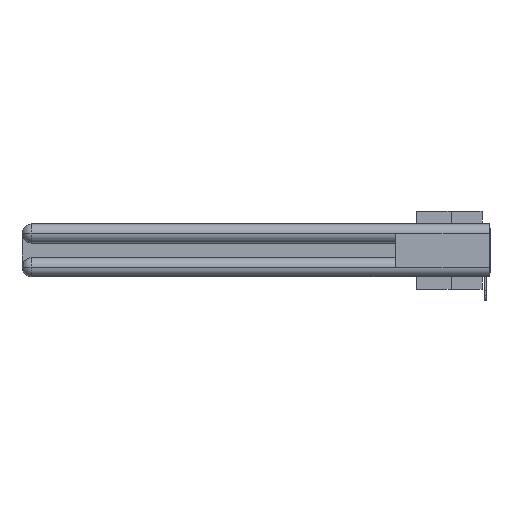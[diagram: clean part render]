
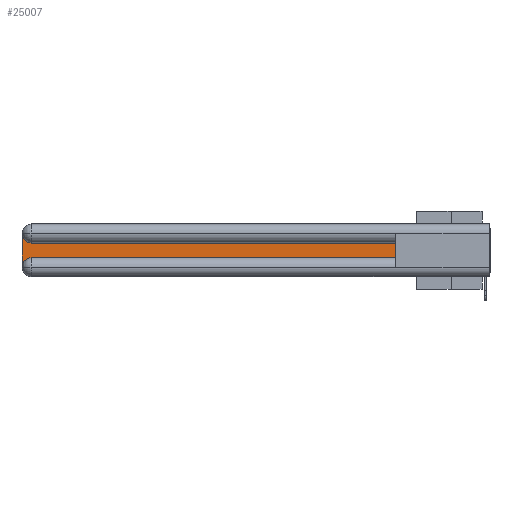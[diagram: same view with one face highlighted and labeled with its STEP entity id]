
A CAD part, left-side view. The second image highlights one B-rep face of the part: STEP entity #25007.
In plain terms, the highlighted planar face has unit normal (-1, 0, 0).
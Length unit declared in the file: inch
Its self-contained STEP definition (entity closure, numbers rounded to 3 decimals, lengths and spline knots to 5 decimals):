
#754 = VECTOR ( 'NONE', #11253, 39.37008 ) ;
#783 = CARTESIAN_POINT ( 'NONE',  ( 0.075, 2.94, -0.2775 ) ) ;
#1091 = DIRECTION ( 'NONE',  ( 1., 0., 0. ) ) ;
#2215 = CIRCLE ( 'NONE', #4742, 0.06 ) ;
#2642 = DIRECTION ( 'NONE',  ( 0., 0., -1. ) ) ;
#4244 = CARTESIAN_POINT ( 'NONE',  ( 0.075, 3., -0.2775 ) ) ;
#4317 = AXIS2_PLACEMENT_3D ( 'NONE', #28802, #22322, #26256 ) ;
#4633 = FACE_OUTER_BOUND ( 'NONE', #37557, .T. ) ;
#4742 = AXIS2_PLACEMENT_3D ( 'NONE', #783, #16528, #22424 ) ;
#6839 = CIRCLE ( 'NONE', #4317, 0.06 ) ;
#7514 = CARTESIAN_POINT ( 'NONE',  ( 0.075, 0.6, -0.2175 ) ) ;
#7869 = ORIENTED_EDGE ( 'NONE', *, *, #36428, .T. ) ;
#8176 = LINE ( 'NONE', #35299, #35453 ) ;
#9497 = EDGE_CURVE ( 'NONE', #30704, #27272, #8176, .T. ) ;
#10113 = CARTESIAN_POINT ( 'NONE',  ( 0.075, 3., -0.0625 ) ) ;
#11253 = DIRECTION ( 'NONE',  ( 0., -1., 0. ) ) ;
#13898 = ORIENTED_EDGE ( 'NONE', *, *, #14002, .T. ) ;
#14002 = EDGE_CURVE ( 'NONE', #16857, #33479, #38190, .T. ) ;
#15342 = VECTOR ( 'NONE', #20244, 39.37008 ) ;
#15763 = VERTEX_POINT ( 'NONE', #17987 ) ;
#16107 = ORIENTED_EDGE ( 'NONE', *, *, #9497, .T. ) ;
#16280 = CARTESIAN_POINT ( 'NONE',  ( 0.075, 0.6, -0.1225 ) ) ;
#16528 = DIRECTION ( 'NONE',  ( 1., 0., 0. ) ) ;
#16857 = VERTEX_POINT ( 'NONE', #19820 ) ;
#17987 = CARTESIAN_POINT ( 'NONE',  ( 0.075, 2.94, -0.1225 ) ) ;
#18820 = ORIENTED_EDGE ( 'NONE', *, *, #37572, .T. ) ;
#19820 = CARTESIAN_POINT ( 'NONE',  ( 0.075, 2.94, -0.2175 ) ) ;
#20244 = DIRECTION ( 'NONE',  ( 0., 0., 1. ) ) ;
#21172 = EDGE_CURVE ( 'NONE', #28078, #15763, #31780, .T. ) ;
#22322 = DIRECTION ( 'NONE',  ( 1., 0., 0. ) ) ;
#22424 = DIRECTION ( 'NONE',  ( 0., 0., -1. ) ) ;
#22997 = CARTESIAN_POINT ( 'NONE',  ( 0.075, 0.6, -0.2175 ) ) ;
#24593 = CARTESIAN_POINT ( 'NONE',  ( 0.075, 0.6, -0.1225 ) ) ;
#25007 = ADVANCED_FACE ( 'NONE', ( #4633 ), #25468, .F. ) ;
#25468 = PLANE ( 'NONE',  #28139 ) ;
#26256 = DIRECTION ( 'NONE',  ( 0., 0., -1. ) ) ;
#26848 = VECTOR ( 'NONE', #31000, 39.37008 ) ;
#27272 = VERTEX_POINT ( 'NONE', #4244 ) ;
#27299 = EDGE_CURVE ( 'NONE', #15763, #30704, #6839, .T. ) ;
#28078 = VERTEX_POINT ( 'NONE', #24593 ) ;
#28139 = AXIS2_PLACEMENT_3D ( 'NONE', #37663, #1091, #34332 ) ;
#28802 = CARTESIAN_POINT ( 'NONE',  ( 0.075, 2.94, -0.0625 ) ) ;
#30704 = VERTEX_POINT ( 'NONE', #10113 ) ;
#31000 = DIRECTION ( 'NONE',  ( 0., 1., 0. ) ) ;
#31780 = LINE ( 'NONE', #16280, #26848 ) ;
#33479 = VERTEX_POINT ( 'NONE', #36456 ) ;
#34332 = DIRECTION ( 'NONE',  ( 0., 0., -1. ) ) ;
#35299 = CARTESIAN_POINT ( 'NONE',  ( 0.075, 3., -0.2175 ) ) ;
#35453 = VECTOR ( 'NONE', #2642, 39.37008 ) ;
#36428 = EDGE_CURVE ( 'NONE', #33479, #28078, #37739, .T. ) ;
#36456 = CARTESIAN_POINT ( 'NONE',  ( 0.075, 0.6, -0.2175 ) ) ;
#37557 = EDGE_LOOP ( 'NONE', ( #38314, #37998, #16107, #18820, #13898, #7869 ) ) ;
#37572 = EDGE_CURVE ( 'NONE', #27272, #16857, #2215, .T. ) ;
#37663 = CARTESIAN_POINT ( 'NONE',  ( 0.075, 3., -0.1225 ) ) ;
#37739 = LINE ( 'NONE', #22997, #15342 ) ;
#37998 = ORIENTED_EDGE ( 'NONE', *, *, #27299, .T. ) ;
#38190 = LINE ( 'NONE', #7514, #754 ) ;
#38314 = ORIENTED_EDGE ( 'NONE', *, *, #21172, .T. ) ;
